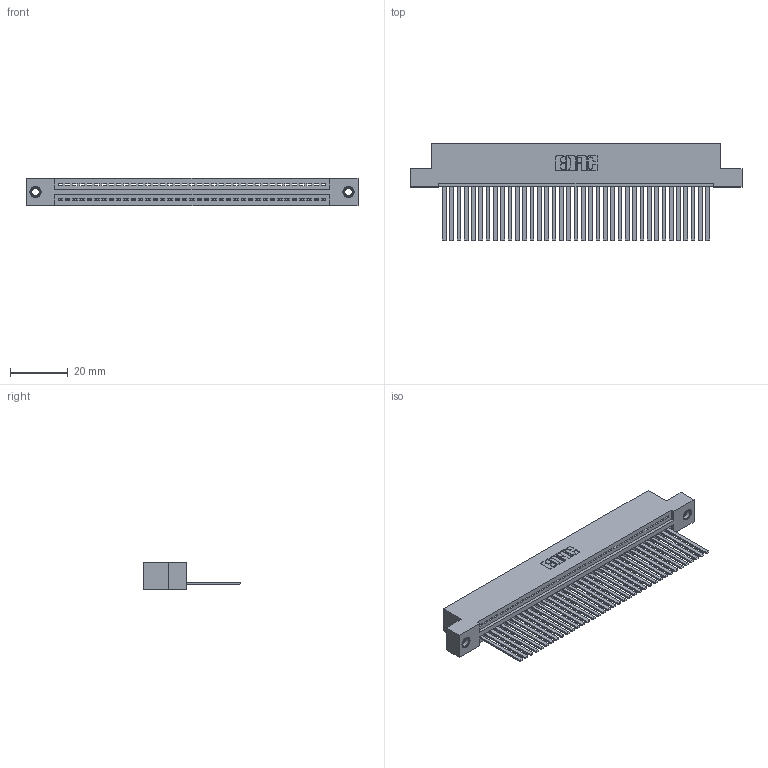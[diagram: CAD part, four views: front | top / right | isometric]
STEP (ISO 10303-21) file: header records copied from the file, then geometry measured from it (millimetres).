
FILE_DESCRIPTION (( 'STEP AP203' ), '1' );
FILE_NAME ('345-037-544-107.STEP', '2018-08-30T03:45:23', ( '' ), ( '' ), 'SwSTEP 2.0', 'SolidWorks 2016', '' );
FILE_SCHEMA (( 'CONFIG_CONTROL_DESIGN' ));
Length unit declared in the file: inch
Products named in the file (4): 345 Part_Flush Mounting Lugs - 0.156 Dia-TI; 345-292-001_345-293-144; 345-250-001_345-250-005-103; 345-037-544-107
Assembly tree (40 placements, depth 2):
  345-037-544-107
    345 Part_Flush Mounting Lugs - 0.156 Dia-TI
    345-292-001_345-293-144  x37
    345-250-001_345-250-005-103  x2
Bounding box: 115.19 x 33.96 x 9.4 mm (x, y, z)
Volume: 11314.8 mm3; surface area: 16287.4 mm2
Topology: 40 solids, 40 shells, 2110 faces, 6323 edges, 4158 vertices
Faces by surface type: plane 1444, cylinder 650, cone 12, torus 4
Entity records: 29522 total; most frequent: CARTESIAN_POINT 5094, ORIENTED_EDGE 5058, DIRECTION 4481, EDGE_CURVE 2529, VECTOR 2233, LINE 2233, VERTEX_POINT 1680, AXIS2_PLACEMENT_3D 1124
